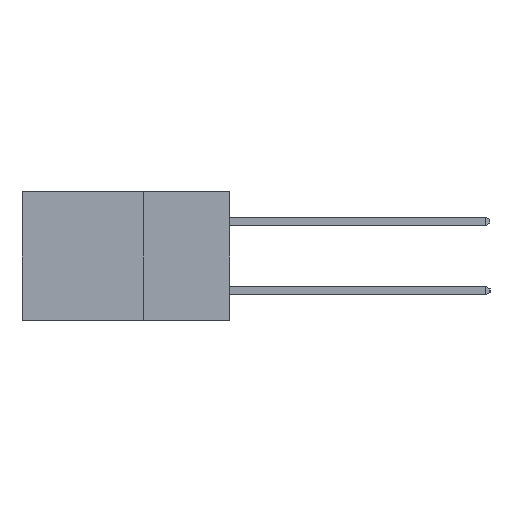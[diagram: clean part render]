
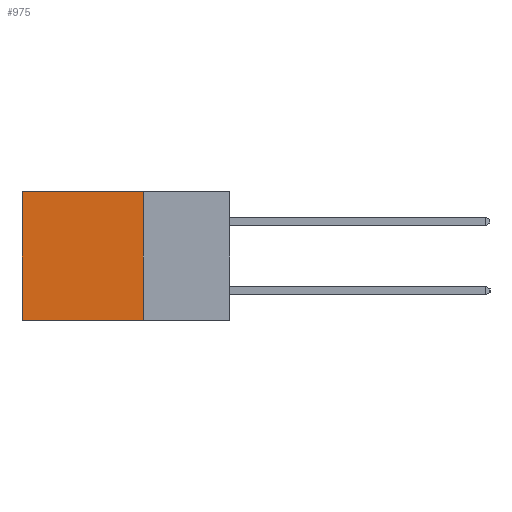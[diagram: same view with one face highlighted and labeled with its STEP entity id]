
A CAD part, left-side view. The second image highlights one B-rep face of the part: STEP entity #975.
In plain terms, the highlighted planar face has unit normal (-1, 0, 0).
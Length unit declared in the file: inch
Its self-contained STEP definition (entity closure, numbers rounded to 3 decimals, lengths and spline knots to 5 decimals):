
#975 = ADVANCED_FACE ( 'NONE', ( #6402 ), #16174, .F. ) ;
#1389 = VERTEX_POINT ( 'NONE', #19009 ) ;
#1410 = CARTESIAN_POINT ( 'NONE',  ( 0.2615, 0.25, -0.37 ) ) ;
#1421 = EDGE_LOOP ( 'NONE', ( #18367, #15006, #18063, #14879 ) ) ;
#1585 = LINE ( 'NONE', #1410, #17578 ) ;
#2271 = VECTOR ( 'NONE', #13503, 39.37008 ) ;
#2727 = CARTESIAN_POINT ( 'NONE',  ( 0.2615, 0.25, 0. ) ) ;
#3349 = VERTEX_POINT ( 'NONE', #2727 ) ;
#3381 = CARTESIAN_POINT ( 'NONE',  ( 0.2615, 0.6, -0.37 ) ) ;
#3467 = EDGE_CURVE ( 'NONE', #3349, #4743, #1585, .T. ) ;
#3632 = EDGE_CURVE ( 'NONE', #1389, #14482, #11103, .T. ) ;
#3962 = VECTOR ( 'NONE', #4442, 39.37008 ) ;
#4442 = DIRECTION ( 'NONE',  ( 0., 1., 0. ) ) ;
#4743 = VERTEX_POINT ( 'NONE', #18204 ) ;
#6038 = CARTESIAN_POINT ( 'NONE',  ( 0.2615, 0.25, 0. ) ) ;
#6124 = EDGE_CURVE ( 'NONE', #4743, #14482, #17737, .T. ) ;
#6232 = EDGE_CURVE ( 'NONE', #3349, #1389, #8625, .T. ) ;
#6402 = FACE_OUTER_BOUND ( 'NONE', #1421, .T. ) ;
#8625 = LINE ( 'NONE', #6038, #3962 ) ;
#9739 = AXIS2_PLACEMENT_3D ( 'NONE', #16042, #15977, #15931 ) ;
#11103 = LINE ( 'NONE', #12635, #14703 ) ;
#11976 = CARTESIAN_POINT ( 'NONE',  ( 0.2615, 0.25, -0.37 ) ) ;
#12300 = DIRECTION ( 'NONE',  ( 0., 0., -1. ) ) ;
#12635 = CARTESIAN_POINT ( 'NONE',  ( 0.2615, 0.6, -0.37 ) ) ;
#12701 = DIRECTION ( 'NONE',  ( 0., 0., -1. ) ) ;
#13503 = DIRECTION ( 'NONE',  ( 0., 1., 0. ) ) ;
#14482 = VERTEX_POINT ( 'NONE', #3381 ) ;
#14703 = VECTOR ( 'NONE', #12701, 39.37008 ) ;
#14879 = ORIENTED_EDGE ( 'NONE', *, *, #6232, .T. ) ;
#15006 = ORIENTED_EDGE ( 'NONE', *, *, #6124, .F. ) ;
#15931 = DIRECTION ( 'NONE',  ( 0., 0., -1. ) ) ;
#15977 = DIRECTION ( 'NONE',  ( 1., 0., 0. ) ) ;
#16042 = CARTESIAN_POINT ( 'NONE',  ( 0.2615, 0.25, -0.37 ) ) ;
#16174 = PLANE ( 'NONE',  #9739 ) ;
#17578 = VECTOR ( 'NONE', #12300, 39.37008 ) ;
#17737 = LINE ( 'NONE', #11976, #2271 ) ;
#18063 = ORIENTED_EDGE ( 'NONE', *, *, #3467, .F. ) ;
#18204 = CARTESIAN_POINT ( 'NONE',  ( 0.2615, 0.25, -0.37 ) ) ;
#18367 = ORIENTED_EDGE ( 'NONE', *, *, #3632, .T. ) ;
#19009 = CARTESIAN_POINT ( 'NONE',  ( 0.2615, 0.6, 0. ) ) ;
